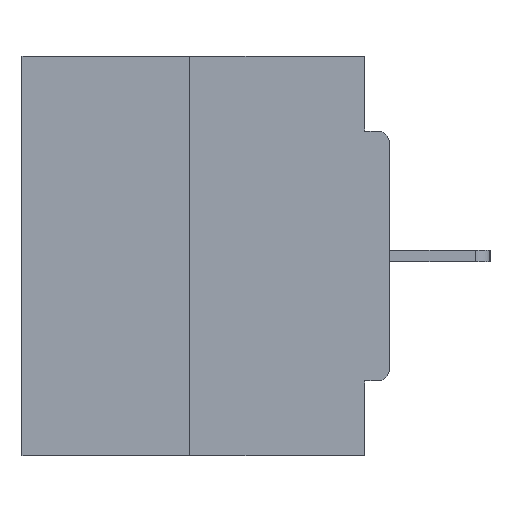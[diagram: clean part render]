
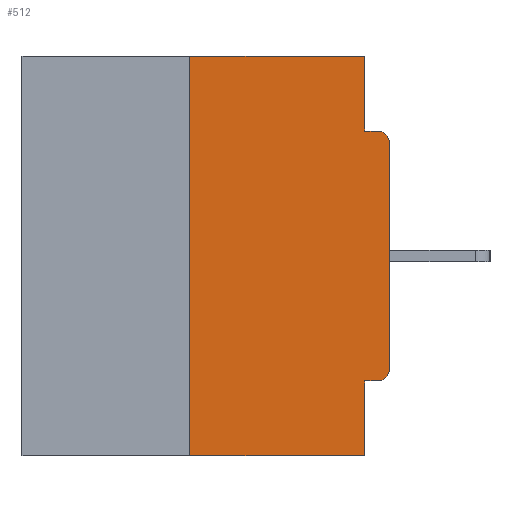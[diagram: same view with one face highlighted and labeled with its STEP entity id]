
A CAD part, left-side view. The second image highlights one B-rep face of the part: STEP entity #512.
In plain terms, the highlighted planar face has unit normal (-1, 0, 0).
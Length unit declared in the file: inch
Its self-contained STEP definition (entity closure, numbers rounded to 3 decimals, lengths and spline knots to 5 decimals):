
#375 = EDGE_CURVE ( 'NONE', #7261, #31942, #2036, .T. ) ;
#417 = ORIENTED_EDGE ( 'NONE', *, *, #33135, .T. ) ;
#512 = ADVANCED_FACE ( 'NONE', ( #12821 ), #36991, .F. ) ;
#1351 = CARTESIAN_POINT ( 'NONE',  ( 0., 0.031, -0.5 ) ) ;
#1591 = EDGE_CURVE ( 'NONE', #23211, #38555, #12086, .T. ) ;
#1768 = CARTESIAN_POINT ( 'NONE',  ( 0., 0.031, -0.5 ) ) ;
#2036 = LINE ( 'NONE', #16925, #25865 ) ;
#2649 = VERTEX_POINT ( 'NONE', #1768 ) ;
#2818 = VERTEX_POINT ( 'NONE', #23259 ) ;
#3861 = ORIENTED_EDGE ( 'NONE', *, *, #1591, .T. ) ;
#4141 = CARTESIAN_POINT ( 'NONE',  ( 0., 0.015, -0.4065 ) ) ;
#4618 = AXIS2_PLACEMENT_3D ( 'NONE', #8200, #29739, #11341 ) ;
#4842 = VERTEX_POINT ( 'NONE', #36071 ) ;
#5369 = VECTOR ( 'NONE', #7077, 39.37008 ) ;
#6198 = ORIENTED_EDGE ( 'NONE', *, *, #38371, .F. ) ;
#6807 = CARTESIAN_POINT ( 'NONE',  ( 0., 0.031, 0. ) ) ;
#6815 = VECTOR ( 'NONE', #18244, 39.37008 ) ;
#7077 = DIRECTION ( 'NONE',  ( 0., -1., 0. ) ) ;
#7261 = VERTEX_POINT ( 'NONE', #6807 ) ;
#7549 = EDGE_CURVE ( 'NONE', #38555, #4842, #8233, .T. ) ;
#8200 = CARTESIAN_POINT ( 'NONE',  ( 0., 0.015, -0.1085 ) ) ;
#8212 = AXIS2_PLACEMENT_3D ( 'NONE', #24877, #22003, #22178 ) ;
#8233 = LINE ( 'NONE', #23260, #15475 ) ;
#10336 = CARTESIAN_POINT ( 'NONE',  ( 0., 0.46, 0. ) ) ;
#11080 = CIRCLE ( 'NONE', #4618, 0.015 ) ;
#11341 = DIRECTION ( 'NONE',  ( 0., 0., -1. ) ) ;
#12086 = CIRCLE ( 'NONE', #8212, 0.015 ) ;
#12100 = CARTESIAN_POINT ( 'NONE',  ( 0., 0., -0.0935 ) ) ;
#12344 = CARTESIAN_POINT ( 'NONE',  ( 0., 0.25, 0. ) ) ;
#12821 = FACE_OUTER_BOUND ( 'NONE', #15948, .T. ) ;
#13482 = VECTOR ( 'NONE', #39035, 39.37008 ) ;
#13683 = LINE ( 'NONE', #31719, #5369 ) ;
#14573 = EDGE_CURVE ( 'NONE', #23211, #2818, #20725, .T. ) ;
#15475 = VECTOR ( 'NONE', #28898, 39.37008 ) ;
#15948 = EDGE_LOOP ( 'NONE', ( #23474, #38498, #417, #30810, #16820, #3861, #31439, #31596, #6198, #30216 ) ) ;
#16820 = ORIENTED_EDGE ( 'NONE', *, *, #14573, .F. ) ;
#16925 = CARTESIAN_POINT ( 'NONE',  ( 0., 0.031, 0. ) ) ;
#17024 = DIRECTION ( 'NONE',  ( 0., 0., -1. ) ) ;
#17465 = AXIS2_PLACEMENT_3D ( 'NONE', #10336, #19701, #24889 ) ;
#17648 = CARTESIAN_POINT ( 'NONE',  ( 0., 0., -0.4065 ) ) ;
#18130 = LINE ( 'NONE', #12344, #24421 ) ;
#18244 = DIRECTION ( 'NONE',  ( 0., -1., 0. ) ) ;
#19701 = DIRECTION ( 'NONE',  ( 1., 0., 0. ) ) ;
#20036 = DIRECTION ( 'NONE',  ( 0., 0., -1. ) ) ;
#20691 = VERTEX_POINT ( 'NONE', #20989 ) ;
#20725 = LINE ( 'NONE', #17648, #13482 ) ;
#20940 = CARTESIAN_POINT ( 'NONE',  ( 0., 0.031, -0.0935 ) ) ;
#20989 = CARTESIAN_POINT ( 'NONE',  ( 0., 0.25, 0. ) ) ;
#21446 = EDGE_CURVE ( 'NONE', #2818, #2649, #33141, .T. ) ;
#22003 = DIRECTION ( 'NONE',  ( -1., 0., 0. ) ) ;
#22178 = DIRECTION ( 'NONE',  ( 0., 0., -1. ) ) ;
#23211 = VERTEX_POINT ( 'NONE', #4141 ) ;
#23259 = CARTESIAN_POINT ( 'NONE',  ( 0., 0.031, -0.4065 ) ) ;
#23260 = CARTESIAN_POINT ( 'NONE',  ( 0., 0., 0. ) ) ;
#23474 = ORIENTED_EDGE ( 'NONE', *, *, #27129, .F. ) ;
#23616 = EDGE_CURVE ( 'NONE', #36998, #20691, #18130, .T. ) ;
#23960 = DIRECTION ( 'NONE',  ( 0., -1., 0. ) ) ;
#24421 = VECTOR ( 'NONE', #36817, 39.37008 ) ;
#24877 = CARTESIAN_POINT ( 'NONE',  ( 0., 0.015, -0.3915 ) ) ;
#24889 = DIRECTION ( 'NONE',  ( 0., 0., -1. ) ) ;
#25865 = VECTOR ( 'NONE', #17024, 39.37008 ) ;
#26478 = VERTEX_POINT ( 'NONE', #33423 ) ;
#27021 = CARTESIAN_POINT ( 'NONE',  ( 0., 0.46, -0.5 ) ) ;
#27129 = EDGE_CURVE ( 'NONE', #20691, #7261, #13683, .T. ) ;
#28898 = DIRECTION ( 'NONE',  ( 0., 0., 1. ) ) ;
#29739 = DIRECTION ( 'NONE',  ( -1., 0., 0. ) ) ;
#30216 = ORIENTED_EDGE ( 'NONE', *, *, #375, .F. ) ;
#30453 = CARTESIAN_POINT ( 'NONE',  ( 0., 0.25, -0.5 ) ) ;
#30810 = ORIENTED_EDGE ( 'NONE', *, *, #21446, .F. ) ;
#31387 = LINE ( 'NONE', #12100, #6815 ) ;
#31439 = ORIENTED_EDGE ( 'NONE', *, *, #7549, .T. ) ;
#31596 = ORIENTED_EDGE ( 'NONE', *, *, #34340, .T. ) ;
#31719 = CARTESIAN_POINT ( 'NONE',  ( 0., 0.46, 0. ) ) ;
#31942 = VERTEX_POINT ( 'NONE', #20940 ) ;
#32195 = VECTOR ( 'NONE', #20036, 39.37008 ) ;
#33135 = EDGE_CURVE ( 'NONE', #36998, #2649, #34679, .T. ) ;
#33141 = LINE ( 'NONE', #1351, #32195 ) ;
#33423 = CARTESIAN_POINT ( 'NONE',  ( 0., 0.015, -0.0935 ) ) ;
#34340 = EDGE_CURVE ( 'NONE', #4842, #26478, #11080, .T. ) ;
#34451 = CARTESIAN_POINT ( 'NONE',  ( 0., 0., -0.3915 ) ) ;
#34679 = LINE ( 'NONE', #27021, #39843 ) ;
#36071 = CARTESIAN_POINT ( 'NONE',  ( 0., 0., -0.1085 ) ) ;
#36817 = DIRECTION ( 'NONE',  ( 0., 0., 1. ) ) ;
#36991 = PLANE ( 'NONE',  #17465 ) ;
#36998 = VERTEX_POINT ( 'NONE', #30453 ) ;
#38371 = EDGE_CURVE ( 'NONE', #31942, #26478, #31387, .T. ) ;
#38498 = ORIENTED_EDGE ( 'NONE', *, *, #23616, .F. ) ;
#38555 = VERTEX_POINT ( 'NONE', #34451 ) ;
#39035 = DIRECTION ( 'NONE',  ( 0., 1., 0. ) ) ;
#39843 = VECTOR ( 'NONE', #23960, 39.37008 ) ;
